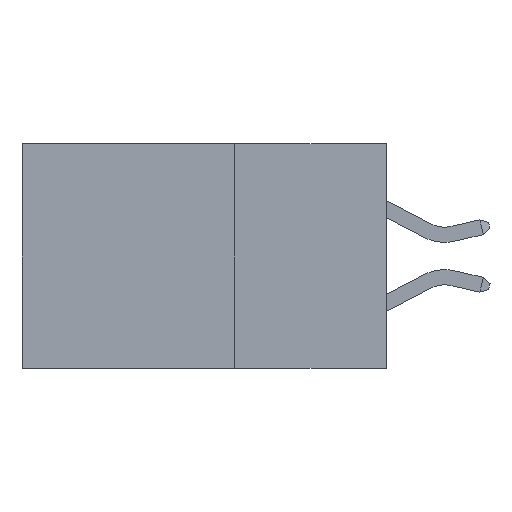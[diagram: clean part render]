
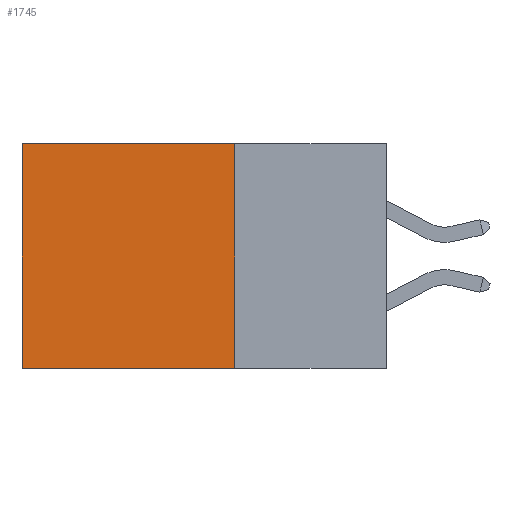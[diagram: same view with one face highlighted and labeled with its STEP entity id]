
A CAD part, left-side view. The second image highlights one B-rep face of the part: STEP entity #1745.
In plain terms, the highlighted planar face has unit normal (-1, 0, 0).
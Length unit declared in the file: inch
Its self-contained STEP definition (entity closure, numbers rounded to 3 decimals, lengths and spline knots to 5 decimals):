
#108 = EDGE_CURVE ( 'NONE', #6308, #6989, #8024, .T. ) ;
#204 = LINE ( 'NONE', #11253, #3780 ) ;
#683 = DIRECTION ( 'NONE',  ( 0., 0., -1. ) ) ;
#1107 = VECTOR ( 'NONE', #9985, 39.37008 ) ;
#1122 = CARTESIAN_POINT ( 'NONE',  ( 0.2615, 0.6, -0.37 ) ) ;
#1691 = ORIENTED_EDGE ( 'NONE', *, *, #11715, .T. ) ;
#1745 = ADVANCED_FACE ( 'NONE', ( #11111 ), #11138, .F. ) ;
#3129 = VECTOR ( 'NONE', #3752, 39.37008 ) ;
#3404 = CARTESIAN_POINT ( 'NONE',  ( 0.2615, 0.6, 0. ) ) ;
#3752 = DIRECTION ( 'NONE',  ( 0., 1., 0. ) ) ;
#3780 = VECTOR ( 'NONE', #6183, 39.37008 ) ;
#4521 = ORIENTED_EDGE ( 'NONE', *, *, #108, .F. ) ;
#6183 = DIRECTION ( 'NONE',  ( 0., 0., -1. ) ) ;
#6222 = AXIS2_PLACEMENT_3D ( 'NONE', #8333, #10745, #12056 ) ;
#6308 = VERTEX_POINT ( 'NONE', #8612 ) ;
#6313 = ORIENTED_EDGE ( 'NONE', *, *, #10978, .F. ) ;
#6768 = LINE ( 'NONE', #1122, #15961 ) ;
#6906 = ORIENTED_EDGE ( 'NONE', *, *, #9789, .T. ) ;
#6989 = VERTEX_POINT ( 'NONE', #13679 ) ;
#8024 = LINE ( 'NONE', #15388, #1107 ) ;
#8063 = CARTESIAN_POINT ( 'NONE',  ( 0.2615, 0.25, 0. ) ) ;
#8333 = CARTESIAN_POINT ( 'NONE',  ( 0.2615, 0.25, -0.37 ) ) ;
#8612 = CARTESIAN_POINT ( 'NONE',  ( 0.2615, 0.25, -0.37 ) ) ;
#9789 = EDGE_CURVE ( 'NONE', #15750, #6989, #6768, .T. ) ;
#9985 = DIRECTION ( 'NONE',  ( 0., 1., 0. ) ) ;
#10302 = LINE ( 'NONE', #11337, #3129 ) ;
#10745 = DIRECTION ( 'NONE',  ( 1., 0., 0. ) ) ;
#10978 = EDGE_CURVE ( 'NONE', #14285, #6308, #204, .T. ) ;
#11111 = FACE_OUTER_BOUND ( 'NONE', #14554, .T. ) ;
#11138 = PLANE ( 'NONE',  #6222 ) ;
#11253 = CARTESIAN_POINT ( 'NONE',  ( 0.2615, 0.25, -0.37 ) ) ;
#11337 = CARTESIAN_POINT ( 'NONE',  ( 0.2615, 0.25, 0. ) ) ;
#11715 = EDGE_CURVE ( 'NONE', #14285, #15750, #10302, .T. ) ;
#12056 = DIRECTION ( 'NONE',  ( 0., 0., -1. ) ) ;
#13679 = CARTESIAN_POINT ( 'NONE',  ( 0.2615, 0.6, -0.37 ) ) ;
#14285 = VERTEX_POINT ( 'NONE', #8063 ) ;
#14554 = EDGE_LOOP ( 'NONE', ( #6906, #4521, #6313, #1691 ) ) ;
#15388 = CARTESIAN_POINT ( 'NONE',  ( 0.2615, 0.25, -0.37 ) ) ;
#15750 = VERTEX_POINT ( 'NONE', #3404 ) ;
#15961 = VECTOR ( 'NONE', #683, 39.37008 ) ;
